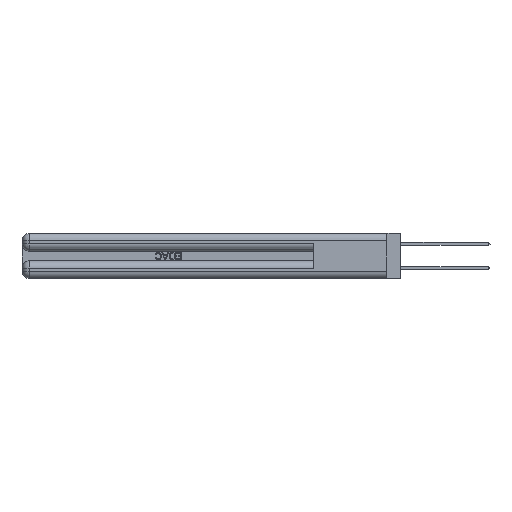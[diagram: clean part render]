
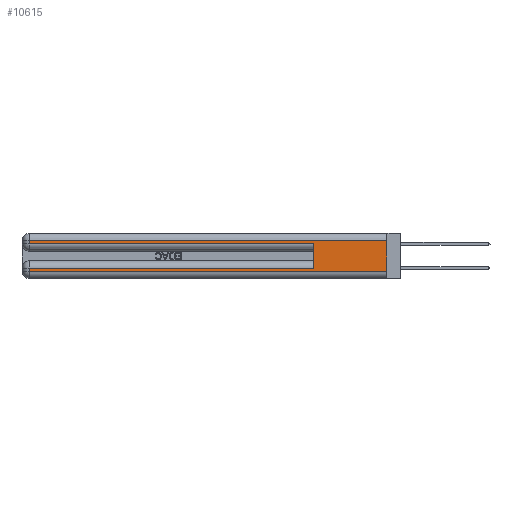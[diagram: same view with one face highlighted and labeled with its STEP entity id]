
A CAD part, left-side view. The second image highlights one B-rep face of the part: STEP entity #10615.
In plain terms, the highlighted planar face has unit normal (-1, 0, 0).
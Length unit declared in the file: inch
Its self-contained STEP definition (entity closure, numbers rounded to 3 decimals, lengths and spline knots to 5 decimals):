
#76 = VECTOR ( 'NONE', #1418, 39.37008 ) ;
#629 = ORIENTED_EDGE ( 'NONE', *, *, #4299, .T. ) ;
#1193 = EDGE_CURVE ( 'NONE', #6884, #21840, #33958, .T. ) ;
#1418 = DIRECTION ( 'NONE',  ( 0., 0., -1. ) ) ;
#1758 = CARTESIAN_POINT ( 'NONE',  ( 0., 0., 0.37 ) ) ;
#2873 = CARTESIAN_POINT ( 'NONE',  ( 0., 2.94, 0.31 ) ) ;
#3026 = ORIENTED_EDGE ( 'NONE', *, *, #45544, .F. ) ;
#3310 = CARTESIAN_POINT ( 'NONE',  ( 0., 0.6, 0.285 ) ) ;
#3474 = CARTESIAN_POINT ( 'NONE',  ( 0., 2.94, 0.085 ) ) ;
#4299 = EDGE_CURVE ( 'NONE', #6884, #27422, #36774, .T. ) ;
#4970 = VERTEX_POINT ( 'NONE', #26366 ) ;
#5789 = DIRECTION ( 'NONE',  ( 0., 1., 0. ) ) ;
#6884 = VERTEX_POINT ( 'NONE', #13539 ) ;
#7373 = CARTESIAN_POINT ( 'NONE',  ( 0., 2.94, 0.37 ) ) ;
#8099 = ORIENTED_EDGE ( 'NONE', *, *, #41622, .T. ) ;
#9801 = DIRECTION ( 'NONE',  ( 0., 1., 0. ) ) ;
#10615 = ADVANCED_FACE ( 'NONE', ( #30209 ), #26680, .F. ) ;
#11205 = CARTESIAN_POINT ( 'NONE',  ( 0., 2.94, 0.37 ) ) ;
#12575 = CARTESIAN_POINT ( 'NONE',  ( 0., 2.94, 0.06 ) ) ;
#12832 = LINE ( 'NONE', #7373, #23480 ) ;
#13539 = CARTESIAN_POINT ( 'NONE',  ( 0., 0., 0.31 ) ) ;
#14459 = LINE ( 'NONE', #37098, #30117 ) ;
#15465 = VECTOR ( 'NONE', #5789, 39.37008 ) ;
#17144 = DIRECTION ( 'NONE',  ( 0., 0., 1. ) ) ;
#18516 = ORIENTED_EDGE ( 'NONE', *, *, #1193, .F. ) ;
#19709 = CARTESIAN_POINT ( 'NONE',  ( 0., 0., 0.285 ) ) ;
#19941 = ORIENTED_EDGE ( 'NONE', *, *, #41938, .T. ) ;
#20980 = CARTESIAN_POINT ( 'NONE',  ( 0., 0., 0.06 ) ) ;
#21493 = LINE ( 'NONE', #19709, #48381 ) ;
#21503 = CARTESIAN_POINT ( 'NONE',  ( 0., 0., 0.085 ) ) ;
#21545 = EDGE_CURVE ( 'NONE', #27422, #33480, #49405, .T. ) ;
#21840 = VERTEX_POINT ( 'NONE', #20980 ) ;
#23480 = VECTOR ( 'NONE', #27815, 39.37008 ) ;
#23753 = DIRECTION ( 'NONE',  ( 0., -1., 0. ) ) ;
#24286 = DIRECTION ( 'NONE',  ( 0., -1., 0. ) ) ;
#24894 = EDGE_LOOP ( 'NONE', ( #18516, #629, #38778, #36254, #3026, #19941, #8099, #26142 ) ) ;
#26142 = ORIENTED_EDGE ( 'NONE', *, *, #48122, .T. ) ;
#26366 = CARTESIAN_POINT ( 'NONE',  ( 0., 0.6, 0.085 ) ) ;
#26680 = PLANE ( 'NONE',  #49764 ) ;
#27422 = VERTEX_POINT ( 'NONE', #2873 ) ;
#27815 = DIRECTION ( 'NONE',  ( 0., 0., -1. ) ) ;
#28188 = VERTEX_POINT ( 'NONE', #12575 ) ;
#29169 = VERTEX_POINT ( 'NONE', #3474 ) ;
#30117 = VECTOR ( 'NONE', #17144, 39.37008 ) ;
#30209 = FACE_OUTER_BOUND ( 'NONE', #24894, .T. ) ;
#30697 = DIRECTION ( 'NONE',  ( 0., 0., -1. ) ) ;
#31153 = DIRECTION ( 'NONE',  ( 0., 0., -1. ) ) ;
#33480 = VERTEX_POINT ( 'NONE', #43550 ) ;
#33958 = LINE ( 'NONE', #1758, #76 ) ;
#33976 = VERTEX_POINT ( 'NONE', #3310 ) ;
#35322 = VECTOR ( 'NONE', #9801, 39.37008 ) ;
#36254 = ORIENTED_EDGE ( 'NONE', *, *, #49961, .T. ) ;
#36772 = LINE ( 'NONE', #47370, #44204 ) ;
#36774 = LINE ( 'NONE', #49491, #15465 ) ;
#37098 = CARTESIAN_POINT ( 'NONE',  ( 0., 0.6, 0.145 ) ) ;
#38753 = DIRECTION ( 'NONE',  ( 1., 0., 0. ) ) ;
#38778 = ORIENTED_EDGE ( 'NONE', *, *, #21545, .T. ) ;
#41622 = EDGE_CURVE ( 'NONE', #29169, #28188, #12832, .T. ) ;
#41938 = EDGE_CURVE ( 'NONE', #4970, #29169, #46604, .T. ) ;
#42528 = VECTOR ( 'NONE', #31153, 39.37008 ) ;
#43550 = CARTESIAN_POINT ( 'NONE',  ( 0., 2.94, 0.285 ) ) ;
#44204 = VECTOR ( 'NONE', #23753, 39.37008 ) ;
#45544 = EDGE_CURVE ( 'NONE', #4970, #33976, #14459, .T. ) ;
#46604 = LINE ( 'NONE', #21503, #35322 ) ;
#47370 = CARTESIAN_POINT ( 'NONE',  ( 0., 0., 0.06 ) ) ;
#48122 = EDGE_CURVE ( 'NONE', #28188, #21840, #36772, .T. ) ;
#48381 = VECTOR ( 'NONE', #24286, 39.37008 ) ;
#49405 = LINE ( 'NONE', #11205, #42528 ) ;
#49491 = CARTESIAN_POINT ( 'NONE',  ( 0., 0., 0.31 ) ) ;
#49764 = AXIS2_PLACEMENT_3D ( 'NONE', #50076, #38753, #30697 ) ;
#49961 = EDGE_CURVE ( 'NONE', #33480, #33976, #21493, .T. ) ;
#50076 = CARTESIAN_POINT ( 'NONE',  ( 0., 0., 0.37 ) ) ;
